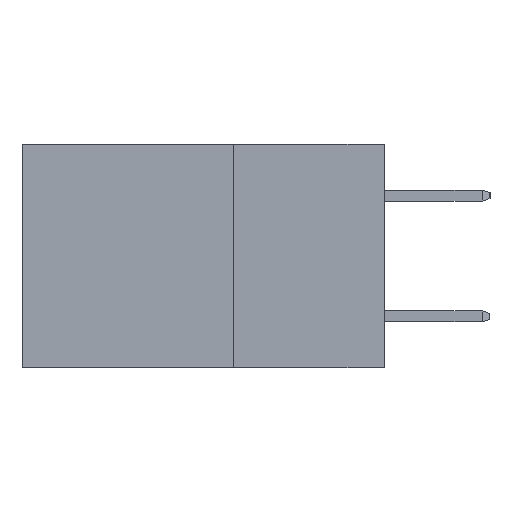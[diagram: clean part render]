
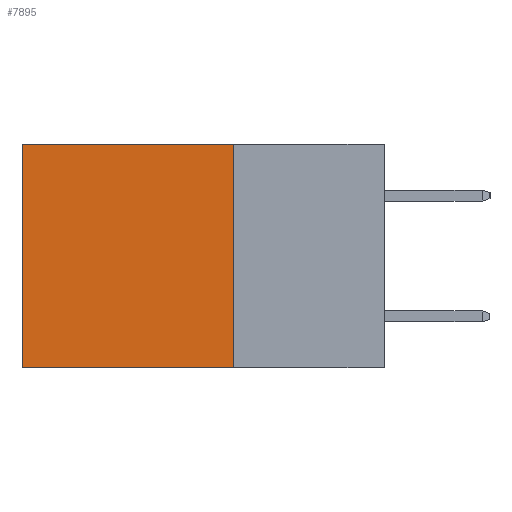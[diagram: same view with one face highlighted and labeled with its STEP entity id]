
A CAD part, left-side view. The second image highlights one B-rep face of the part: STEP entity #7895.
In plain terms, the highlighted planar face has unit normal (-1, 0, 0).
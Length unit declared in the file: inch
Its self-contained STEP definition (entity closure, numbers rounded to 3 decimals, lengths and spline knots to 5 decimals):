
#565 = VECTOR ( 'NONE', #6494, 39.37008 ) ;
#815 = VECTOR ( 'NONE', #15213, 39.37008 ) ;
#1798 = EDGE_CURVE ( 'NONE', #7453, #4520, #14351, .T. ) ;
#1801 = ORIENTED_EDGE ( 'NONE', *, *, #5281, .T. ) ;
#2180 = VECTOR ( 'NONE', #6988, 39.37008 ) ;
#2455 = CARTESIAN_POINT ( 'NONE',  ( 0.298, 0.25, 0. ) ) ;
#2737 = LINE ( 'NONE', #19034, #2180 ) ;
#4520 = VERTEX_POINT ( 'NONE', #17665 ) ;
#5281 = EDGE_CURVE ( 'NONE', #19079, #4520, #2737, .T. ) ;
#5335 = ORIENTED_EDGE ( 'NONE', *, *, #1798, .F. ) ;
#5532 = VECTOR ( 'NONE', #21385, 39.37008 ) ;
#6494 = DIRECTION ( 'NONE',  ( 0., 1., 0. ) ) ;
#6988 = DIRECTION ( 'NONE',  ( 0., 0., -1. ) ) ;
#7088 = EDGE_LOOP ( 'NONE', ( #1801, #5335, #18402, #12940 ) ) ;
#7453 = VERTEX_POINT ( 'NONE', #15845 ) ;
#7895 = ADVANCED_FACE ( 'NONE', ( #14180 ), #17981, .F. ) ;
#9411 = DIRECTION ( 'NONE',  ( 0., 0., -1. ) ) ;
#9447 = CARTESIAN_POINT ( 'NONE',  ( 0.298, 0.25, 0. ) ) ;
#9966 = AXIS2_PLACEMENT_3D ( 'NONE', #2455, #19701, #9411 ) ;
#11310 = EDGE_CURVE ( 'NONE', #15071, #7453, #14129, .T. ) ;
#12940 = ORIENTED_EDGE ( 'NONE', *, *, #21439, .T. ) ;
#13475 = CARTESIAN_POINT ( 'NONE',  ( 0.298, 0.25, 0. ) ) ;
#14129 = LINE ( 'NONE', #9447, #5532 ) ;
#14180 = FACE_OUTER_BOUND ( 'NONE', #7088, .T. ) ;
#14351 = LINE ( 'NONE', #17075, #565 ) ;
#15071 = VERTEX_POINT ( 'NONE', #20335 ) ;
#15213 = DIRECTION ( 'NONE',  ( 0., 1., 0. ) ) ;
#15845 = CARTESIAN_POINT ( 'NONE',  ( 0.298, 0.25, -0.37 ) ) ;
#17075 = CARTESIAN_POINT ( 'NONE',  ( 0.298, 0.25, -0.37 ) ) ;
#17665 = CARTESIAN_POINT ( 'NONE',  ( 0.298, 0.6, -0.37 ) ) ;
#17981 = PLANE ( 'NONE',  #9966 ) ;
#18146 = CARTESIAN_POINT ( 'NONE',  ( 0.298, 0.6, 0. ) ) ;
#18402 = ORIENTED_EDGE ( 'NONE', *, *, #11310, .F. ) ;
#19034 = CARTESIAN_POINT ( 'NONE',  ( 0.298, 0.6, 0. ) ) ;
#19079 = VERTEX_POINT ( 'NONE', #18146 ) ;
#19187 = LINE ( 'NONE', #13475, #815 ) ;
#19701 = DIRECTION ( 'NONE',  ( 1., 0., 0. ) ) ;
#20335 = CARTESIAN_POINT ( 'NONE',  ( 0.298, 0.25, 0. ) ) ;
#21385 = DIRECTION ( 'NONE',  ( 0., 0., -1. ) ) ;
#21439 = EDGE_CURVE ( 'NONE', #15071, #19079, #19187, .T. ) ;
